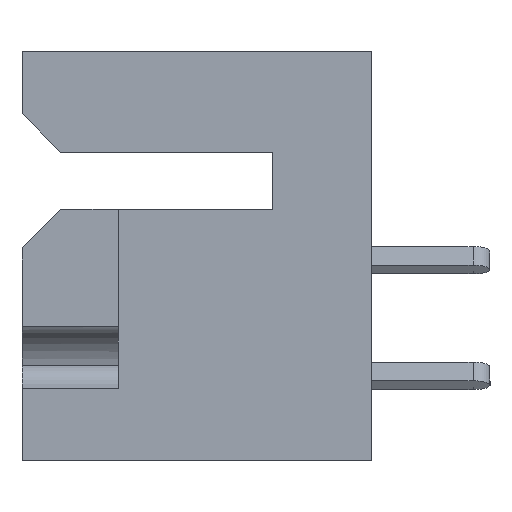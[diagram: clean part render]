
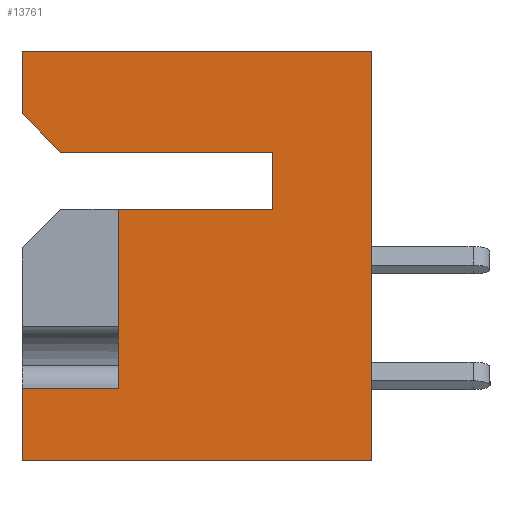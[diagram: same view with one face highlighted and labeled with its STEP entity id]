
A CAD part, left-side view. The second image highlights one B-rep face of the part: STEP entity #13761.
In plain terms, the highlighted planar face has unit normal (-1, 0, 0).
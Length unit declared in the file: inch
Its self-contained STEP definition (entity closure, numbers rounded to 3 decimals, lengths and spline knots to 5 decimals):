
#199 = VECTOR ( 'NONE', #11388, 39.37008 ) ;
#537 = VERTEX_POINT ( 'NONE', #6470 ) ;
#738 = EDGE_CURVE ( 'NONE', #2333, #537, #772, .T. ) ;
#772 = LINE ( 'NONE', #4394, #19059 ) ;
#776 = ORIENTED_EDGE ( 'NONE', *, *, #4836, .F. ) ;
#1488 = EDGE_LOOP ( 'NONE', ( #5941, #776, #7893, #12025, #9209, #13414, #13570, #9100, #9923, #11316, #14863 ) ) ;
#1622 = CARTESIAN_POINT ( 'NONE',  ( 0., 0.453, -0.437 ) ) ;
#1830 = CARTESIAN_POINT ( 'NONE',  ( 0., 0.453, 0. ) ) ;
#2062 = CARTESIAN_POINT ( 'NONE',  ( 0., 0.328, -0.437 ) ) ;
#2333 = VERTEX_POINT ( 'NONE', #5451 ) ;
#2551 = CARTESIAN_POINT ( 'NONE',  ( 0., 0.128, -0.205 ) ) ;
#2594 = DIRECTION ( 'NONE',  ( 0., 0., 1. ) ) ;
#3102 = LINE ( 'NONE', #6417, #15777 ) ;
#3337 = FACE_OUTER_BOUND ( 'NONE', #1488, .T. ) ;
#3478 = CARTESIAN_POINT ( 'NONE',  ( 0., 0.128, -0.205 ) ) ;
#4157 = CARTESIAN_POINT ( 'NONE',  ( 0., 0.328, -0.205 ) ) ;
#4394 = CARTESIAN_POINT ( 'NONE',  ( 0., 0.403, -0.131 ) ) ;
#4836 = EDGE_CURVE ( 'NONE', #11948, #11882, #18228, .T. ) ;
#4860 = VECTOR ( 'NONE', #15056, 39.37008 ) ;
#5184 = DIRECTION ( 'NONE',  ( 0., 0., 1. ) ) ;
#5319 = PLANE ( 'NONE',  #12123 ) ;
#5331 = CARTESIAN_POINT ( 'NONE',  ( 0., 0., 0. ) ) ;
#5423 = VERTEX_POINT ( 'NONE', #21138 ) ;
#5451 = CARTESIAN_POINT ( 'NONE',  ( 0., 0.453, -0.081 ) ) ;
#5458 = VECTOR ( 'NONE', #16249, 39.37008 ) ;
#5941 = ORIENTED_EDGE ( 'NONE', *, *, #15408, .T. ) ;
#6356 = EDGE_CURVE ( 'NONE', #6795, #14616, #22186, .T. ) ;
#6410 = VERTEX_POINT ( 'NONE', #9894 ) ;
#6417 = CARTESIAN_POINT ( 'NONE',  ( 0., 0.453, -0.531 ) ) ;
#6470 = CARTESIAN_POINT ( 'NONE',  ( 0., 0.403, -0.131 ) ) ;
#6795 = VERTEX_POINT ( 'NONE', #2062 ) ;
#7726 = DIRECTION ( 'NONE',  ( 0., -0.707, -0.707 ) ) ;
#7843 = DIRECTION ( 'NONE',  ( 0., 1., 0. ) ) ;
#7893 = ORIENTED_EDGE ( 'NONE', *, *, #12411, .T. ) ;
#7949 = CARTESIAN_POINT ( 'NONE',  ( 0., 0., -0.531 ) ) ;
#8061 = CARTESIAN_POINT ( 'NONE',  ( 0., 0.328, -0.437 ) ) ;
#8766 = VERTEX_POINT ( 'NONE', #3478 ) ;
#9092 = VECTOR ( 'NONE', #13899, 39.37008 ) ;
#9100 = ORIENTED_EDGE ( 'NONE', *, *, #16655, .F. ) ;
#9209 = ORIENTED_EDGE ( 'NONE', *, *, #10761, .F. ) ;
#9336 = VERTEX_POINT ( 'NONE', #20575 ) ;
#9448 = CARTESIAN_POINT ( 'NONE',  ( 0., 0.453, 0. ) ) ;
#9566 = CARTESIAN_POINT ( 'NONE',  ( 0., 0.128, -0.131 ) ) ;
#9894 = CARTESIAN_POINT ( 'NONE',  ( 0., 0.453, 0. ) ) ;
#9923 = ORIENTED_EDGE ( 'NONE', *, *, #18445, .F. ) ;
#9986 = LINE ( 'NONE', #8061, #4860 ) ;
#10374 = VECTOR ( 'NONE', #14662, 39.37008 ) ;
#10440 = CARTESIAN_POINT ( 'NONE',  ( 0., 0.453, -0.531 ) ) ;
#10453 = LINE ( 'NONE', #11481, #16645 ) ;
#10761 = EDGE_CURVE ( 'NONE', #6410, #5423, #19870, .T. ) ;
#11289 = LINE ( 'NONE', #9566, #19335 ) ;
#11316 = ORIENTED_EDGE ( 'NONE', *, *, #20533, .T. ) ;
#11318 = EDGE_CURVE ( 'NONE', #17735, #5423, #21451, .T. ) ;
#11388 = DIRECTION ( 'NONE',  ( 0., 0., 1. ) ) ;
#11481 = CARTESIAN_POINT ( 'NONE',  ( 0., 0.453, 0. ) ) ;
#11505 = LINE ( 'NONE', #13183, #199 ) ;
#11882 = VERTEX_POINT ( 'NONE', #1622 ) ;
#11948 = VERTEX_POINT ( 'NONE', #10440 ) ;
#12025 = ORIENTED_EDGE ( 'NONE', *, *, #11318, .T. ) ;
#12123 = AXIS2_PLACEMENT_3D ( 'NONE', #20747, #17445, #17228 ) ;
#12411 = EDGE_CURVE ( 'NONE', #11948, #17735, #3102, .T. ) ;
#12927 = CARTESIAN_POINT ( 'NONE',  ( 0., 0.328, -0.205 ) ) ;
#13183 = CARTESIAN_POINT ( 'NONE',  ( 0., 0.128, -0.131 ) ) ;
#13398 = VECTOR ( 'NONE', #5184, 39.37008 ) ;
#13414 = ORIENTED_EDGE ( 'NONE', *, *, #17860, .F. ) ;
#13570 = ORIENTED_EDGE ( 'NONE', *, *, #738, .T. ) ;
#13761 = ADVANCED_FACE ( 'NONE', ( #3337 ), #5319, .F. ) ;
#13899 = DIRECTION ( 'NONE',  ( 0., -1., 0. ) ) ;
#14616 = VERTEX_POINT ( 'NONE', #4157 ) ;
#14662 = DIRECTION ( 'NONE',  ( 0., 0., 1. ) ) ;
#14863 = ORIENTED_EDGE ( 'NONE', *, *, #6356, .F. ) ;
#15056 = DIRECTION ( 'NONE',  ( 0., 1., 0. ) ) ;
#15095 = DIRECTION ( 'NONE',  ( 0., 0., 1. ) ) ;
#15408 = EDGE_CURVE ( 'NONE', #6795, #11882, #9986, .T. ) ;
#15706 = LINE ( 'NONE', #2551, #5458 ) ;
#15777 = VECTOR ( 'NONE', #16820, 39.37008 ) ;
#16249 = DIRECTION ( 'NONE',  ( 0., 1., 0. ) ) ;
#16645 = VECTOR ( 'NONE', #15095, 39.37008 ) ;
#16655 = EDGE_CURVE ( 'NONE', #9336, #537, #11289, .T. ) ;
#16820 = DIRECTION ( 'NONE',  ( 0., -1., 0. ) ) ;
#17228 = DIRECTION ( 'NONE',  ( 0., 0., -1. ) ) ;
#17445 = DIRECTION ( 'NONE',  ( 1., 0., 0. ) ) ;
#17735 = VERTEX_POINT ( 'NONE', #7949 ) ;
#17860 = EDGE_CURVE ( 'NONE', #2333, #6410, #10453, .T. ) ;
#18228 = LINE ( 'NONE', #9448, #19834 ) ;
#18445 = EDGE_CURVE ( 'NONE', #8766, #9336, #11505, .T. ) ;
#19059 = VECTOR ( 'NONE', #7726, 39.37008 ) ;
#19335 = VECTOR ( 'NONE', #7843, 39.37008 ) ;
#19834 = VECTOR ( 'NONE', #2594, 39.37008 ) ;
#19870 = LINE ( 'NONE', #1830, #9092 ) ;
#20533 = EDGE_CURVE ( 'NONE', #8766, #14616, #15706, .T. ) ;
#20575 = CARTESIAN_POINT ( 'NONE',  ( 0., 0.128, -0.131 ) ) ;
#20747 = CARTESIAN_POINT ( 'NONE',  ( 0., 0.453, 0. ) ) ;
#21138 = CARTESIAN_POINT ( 'NONE',  ( 0., 0., 0. ) ) ;
#21451 = LINE ( 'NONE', #5331, #13398 ) ;
#22186 = LINE ( 'NONE', #12927, #10374 ) ;
